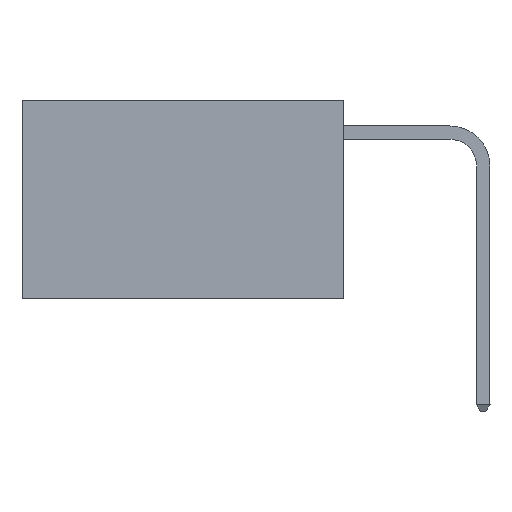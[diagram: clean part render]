
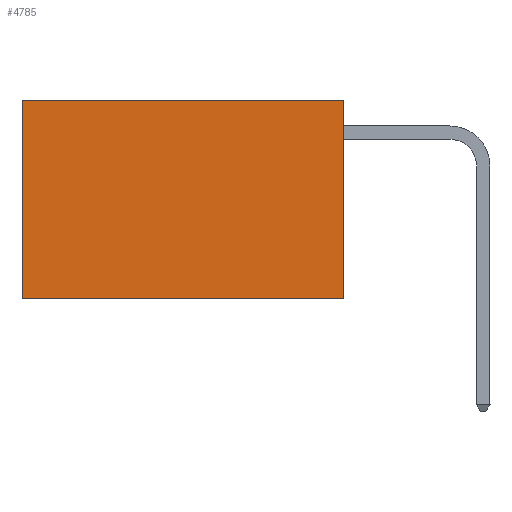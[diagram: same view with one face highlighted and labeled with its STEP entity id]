
A CAD part, left-side view. The second image highlights one B-rep face of the part: STEP entity #4785.
In plain terms, the highlighted planar face has unit normal (-1, 0, 0).
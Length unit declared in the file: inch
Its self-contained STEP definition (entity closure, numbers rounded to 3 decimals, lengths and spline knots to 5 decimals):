
#164 = DIRECTION ( 'NONE',  ( 0., 1., 0. ) ) ;
#1087 = EDGE_CURVE ( 'NONE', #11805, #10691, #1551, .T. ) ;
#1098 = DIRECTION ( 'NONE',  ( 0., 0., -1. ) ) ;
#1220 = ORIENTED_EDGE ( 'NONE', *, *, #10857, .T. ) ;
#1470 = EDGE_LOOP ( 'NONE', ( #2766, #3932, #4413, #1220 ) ) ;
#1551 = LINE ( 'NONE', #6186, #6608 ) ;
#1898 = EDGE_CURVE ( 'NONE', #2469, #11491, #5962, .T. ) ;
#2096 = LINE ( 'NONE', #6736, #7099 ) ;
#2469 = VERTEX_POINT ( 'NONE', #11811 ) ;
#2766 = ORIENTED_EDGE ( 'NONE', *, *, #1087, .T. ) ;
#3380 = VECTOR ( 'NONE', #8215, 39.37008 ) ;
#3932 = ORIENTED_EDGE ( 'NONE', *, *, #4933, .F. ) ;
#4413 = ORIENTED_EDGE ( 'NONE', *, *, #1898, .F. ) ;
#4443 = CARTESIAN_POINT ( 'NONE',  ( 0.2625, 0., -0.37 ) ) ;
#4572 = CARTESIAN_POINT ( 'NONE',  ( 0.2625, 0., 0. ) ) ;
#4785 = ADVANCED_FACE ( 'NONE', ( #9427 ), #8137, .F. ) ;
#4933 = EDGE_CURVE ( 'NONE', #11491, #10691, #7224, .T. ) ;
#5140 = AXIS2_PLACEMENT_3D ( 'NONE', #6187, #7179, #1098 ) ;
#5962 = LINE ( 'NONE', #4572, #3380 ) ;
#6186 = CARTESIAN_POINT ( 'NONE',  ( 0.2625, 0.6, 0. ) ) ;
#6187 = CARTESIAN_POINT ( 'NONE',  ( 0.2625, 0., 0. ) ) ;
#6533 = DIRECTION ( 'NONE',  ( 0., 1., 0. ) ) ;
#6608 = VECTOR ( 'NONE', #6888, 39.37008 ) ;
#6736 = CARTESIAN_POINT ( 'NONE',  ( 0.2625, 0., 0. ) ) ;
#6888 = DIRECTION ( 'NONE',  ( 0., 0., -1. ) ) ;
#7099 = VECTOR ( 'NONE', #6533, 39.37008 ) ;
#7179 = DIRECTION ( 'NONE',  ( 1., 0., 0. ) ) ;
#7224 = LINE ( 'NONE', #4443, #12218 ) ;
#8137 = PLANE ( 'NONE',  #5140 ) ;
#8215 = DIRECTION ( 'NONE',  ( 0., 0., -1. ) ) ;
#9255 = CARTESIAN_POINT ( 'NONE',  ( 0.2625, 0.6, 0. ) ) ;
#9427 = FACE_OUTER_BOUND ( 'NONE', #1470, .T. ) ;
#10691 = VERTEX_POINT ( 'NONE', #12329 ) ;
#10857 = EDGE_CURVE ( 'NONE', #2469, #11805, #2096, .T. ) ;
#11491 = VERTEX_POINT ( 'NONE', #12707 ) ;
#11805 = VERTEX_POINT ( 'NONE', #9255 ) ;
#11811 = CARTESIAN_POINT ( 'NONE',  ( 0.2625, 0., 0. ) ) ;
#12218 = VECTOR ( 'NONE', #164, 39.37008 ) ;
#12329 = CARTESIAN_POINT ( 'NONE',  ( 0.2625, 0.6, -0.37 ) ) ;
#12707 = CARTESIAN_POINT ( 'NONE',  ( 0.2625, 0., -0.37 ) ) ;
